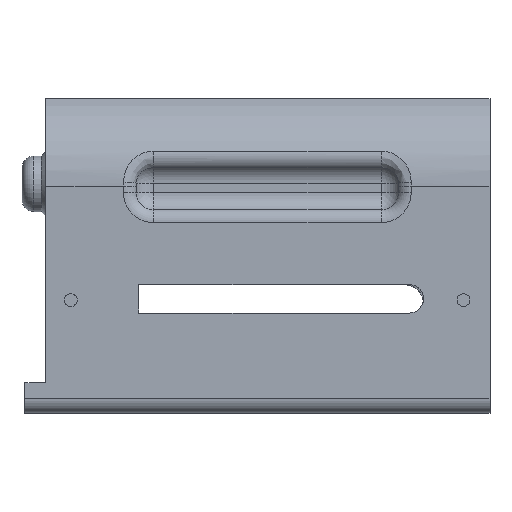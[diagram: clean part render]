
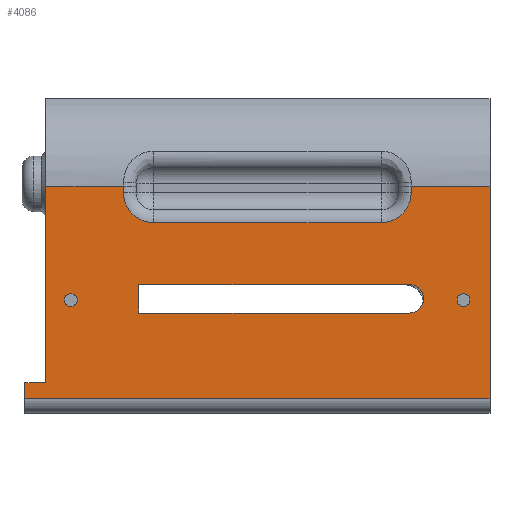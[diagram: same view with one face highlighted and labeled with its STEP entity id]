
A CAD part, top view. The second image highlights one B-rep face of the part: STEP entity #4086.
In plain terms, the highlighted planar face has unit normal (0, 0, 1).
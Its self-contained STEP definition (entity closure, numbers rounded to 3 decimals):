
#24 = ORIENTED_EDGE ( 'NONE', *, *, #6329, .F. ) ;
#39 = CARTESIAN_POINT ( 'NONE',  ( 83.403, 40.151, 20.1 ) ) ;
#65 = AXIS2_PLACEMENT_3D ( 'NONE', #5753, #6270, #804 ) ;
#95 = VERTEX_POINT ( 'NONE', #1609 ) ;
#123 = FACE_BOUND ( 'NONE', #307, .T. ) ;
#135 = LINE ( 'NONE', #2848, #3104 ) ;
#181 = VERTEX_POINT ( 'NONE', #1326 ) ;
#194 = LINE ( 'NONE', #2502, #4265 ) ;
#267 = VECTOR ( 'NONE', #2964, 1000. ) ;
#307 = EDGE_LOOP ( 'NONE', ( #24, #4251, #1701, #4105 ) ) ;
#310 = DIRECTION ( 'NONE',  ( -0.707, -0.707, 0. ) ) ;
#328 = CIRCLE ( 'NONE', #1395, 1.35 ) ;
#372 = EDGE_CURVE ( 'NONE', #4874, #4902, #4618, .T. ) ;
#436 = DIRECTION ( 'NONE',  ( 0., 0., 1. ) ) ;
#480 = CARTESIAN_POINT ( 'NONE',  ( 106.318, 71.272, 20.1 ) ) ;
#500 = VECTOR ( 'NONE', #5597, 1000. ) ;
#507 = CIRCLE ( 'NONE', #65, 6.325 ) ;
#534 = CARTESIAN_POINT ( 'NONE',  ( 17.987, 23.82, 20.1 ) ) ;
#618 = VERTEX_POINT ( 'NONE', #5741 ) ;
#677 = VERTEX_POINT ( 'NONE', #3186 ) ;
#678 = CIRCLE ( 'NONE', #3314, 6.325 ) ;
#804 = DIRECTION ( 'NONE',  ( 0.707, -0.707, 0. ) ) ;
#860 = EDGE_LOOP ( 'NONE', ( #1579 ) ) ;
#869 = CARTESIAN_POINT ( 'NONE',  ( 89.318, 27.078, 20.1 ) ) ;
#918 = EDGE_CURVE ( 'NONE', #4902, #1303, #1089, .T. ) ;
#957 = CARTESIAN_POINT ( 'NONE',  ( 8.3, 3.06, 20.1 ) ) ;
#1036 = DIRECTION ( 'NONE',  ( 0., 0., -1. ) ) ;
#1089 = CIRCLE ( 'NONE', #3141, 3. ) ;
#1100 = EDGE_CURVE ( 'NONE', #5980, #677, #2735, .T. ) ;
#1127 = ORIENTED_EDGE ( 'NONE', *, *, #5812, .T. ) ;
#1143 = VECTOR ( 'NONE', #2233, 1000. ) ;
#1180 = ORIENTED_EDGE ( 'NONE', *, *, #1100, .T. ) ;
#1276 = CARTESIAN_POINT ( 'NONE',  ( 35.403, 46.476, 20.1 ) ) ;
#1278 = VECTOR ( 'NONE', #5903, 1000. ) ;
#1286 = ORIENTED_EDGE ( 'NONE', *, *, #6173, .F. ) ;
#1298 = VERTEX_POINT ( 'NONE', #3364 ) ;
#1300 = CARTESIAN_POINT ( 'NONE',  ( 29.079, 47.476, 20.1 ) ) ;
#1303 = VERTEX_POINT ( 'NONE', #869 ) ;
#1326 = CARTESIAN_POINT ( 'NONE',  ( 16.637, 23.82, 20.1 ) ) ;
#1349 = VECTOR ( 'NONE', #4595, 1000. ) ;
#1395 = AXIS2_PLACEMENT_3D ( 'NONE', #534, #3577, #5480 ) ;
#1575 = DIRECTION ( 'NONE',  ( 0., 1., 0. ) ) ;
#1579 = ORIENTED_EDGE ( 'NONE', *, *, #5364, .T. ) ;
#1609 = CARTESIAN_POINT ( 'NONE',  ( 32.318, 27.078, 20.1 ) ) ;
#1679 = LINE ( 'NONE', #1300, #2920 ) ;
#1701 = ORIENTED_EDGE ( 'NONE', *, *, #918, .F. ) ;
#1733 = CARTESIAN_POINT ( 'NONE',  ( 12.7, 3.06, 20.1 ) ) ;
#1740 = CARTESIAN_POINT ( 'NONE',  ( 12.7, 6.41, 20.1 ) ) ;
#1744 = VERTEX_POINT ( 'NONE', #39 ) ;
#1795 = ORIENTED_EDGE ( 'NONE', *, *, #5772, .F. ) ;
#1825 = LINE ( 'NONE', #1995, #5494 ) ;
#1828 = CARTESIAN_POINT ( 'NONE',  ( 18.04, 47.837, 20.1 ) ) ;
#1995 = CARTESIAN_POINT ( 'NONE',  ( 89.728, 47.476, 20.1 ) ) ;
#2050 = VECTOR ( 'NONE', #5286, 1000. ) ;
#2138 = AXIS2_PLACEMENT_3D ( 'NONE', #6451, #2908, #1575 ) ;
#2212 = LINE ( 'NONE', #1828, #2050 ) ;
#2213 = EDGE_LOOP ( 'NONE', ( #3855 ) ) ;
#2233 = DIRECTION ( 'NONE',  ( -1., 0., 0. ) ) ;
#2243 = CARTESIAN_POINT ( 'NONE',  ( 8.3, 6.41, 20.1 ) ) ;
#2251 = VECTOR ( 'NONE', #3181, 1000. ) ;
#2276 = CARTESIAN_POINT ( 'NONE',  ( 32.318, 21.078, 20.1 ) ) ;
#2292 = CARTESIAN_POINT ( 'NONE',  ( 89.728, 46.476, 20.1 ) ) ;
#2496 = CARTESIAN_POINT ( 'NONE',  ( 32.318, 12.068, 20.1 ) ) ;
#2502 = CARTESIAN_POINT ( 'NONE',  ( 8.3, 45.001, 20.1 ) ) ;
#2638 = EDGE_CURVE ( 'NONE', #1303, #95, #135, .T. ) ;
#2689 = LINE ( 'NONE', #2496, #500 ) ;
#2735 = LINE ( 'NONE', #6049, #2251 ) ;
#2747 = ORIENTED_EDGE ( 'NONE', *, *, #5531, .F. ) ;
#2794 = CARTESIAN_POINT ( 'NONE',  ( 25.408, 21.078, 20.1 ) ) ;
#2820 = EDGE_CURVE ( 'NONE', #3206, #5874, #5272, .T. ) ;
#2835 = DIRECTION ( 'NONE',  ( 0., -1., 0. ) ) ;
#2848 = CARTESIAN_POINT ( 'NONE',  ( 25.408, 27.078, 20.1 ) ) ;
#2851 = LINE ( 'NONE', #480, #267 ) ;
#2908 = DIRECTION ( 'NONE',  ( 0., 0., -1. ) ) ;
#2916 = VERTEX_POINT ( 'NONE', #5376 ) ;
#2920 = VECTOR ( 'NONE', #2835, 1000. ) ;
#2960 = VERTEX_POINT ( 'NONE', #2243 ) ;
#2964 = DIRECTION ( 'NONE',  ( 0., 1., 0. ) ) ;
#3104 = VECTOR ( 'NONE', #4840, 1000. ) ;
#3141 = AXIS2_PLACEMENT_3D ( 'NONE', #4435, #436, #3921 ) ;
#3181 = DIRECTION ( 'NONE',  ( 0., -1., 0. ) ) ;
#3186 = CARTESIAN_POINT ( 'NONE',  ( 12.7, 6.41, 20.1 ) ) ;
#3206 = VERTEX_POINT ( 'NONE', #4051 ) ;
#3314 = AXIS2_PLACEMENT_3D ( 'NONE', #1276, #3316, #310 ) ;
#3316 = DIRECTION ( 'NONE',  ( 0., 0., 1. ) ) ;
#3332 = FACE_OUTER_BOUND ( 'NONE', #3971, .T. ) ;
#3364 = CARTESIAN_POINT ( 'NONE',  ( 35.403, 40.151, 20.1 ) ) ;
#3369 = CARTESIAN_POINT ( 'NONE',  ( 29.079, 47.837, 20.1 ) ) ;
#3406 = CARTESIAN_POINT ( 'NONE',  ( 89.728, 47.837, 20.1 ) ) ;
#3504 = EDGE_CURVE ( 'NONE', #618, #1298, #678, .T. ) ;
#3513 = ORIENTED_EDGE ( 'NONE', *, *, #6301, .F. ) ;
#3577 = DIRECTION ( 'NONE',  ( 0., 0., -1. ) ) ;
#3626 = ORIENTED_EDGE ( 'NONE', *, *, #5834, .T. ) ;
#3688 = CARTESIAN_POINT ( 'NONE',  ( 106.318, 47.837, 20.1 ) ) ;
#3796 = LINE ( 'NONE', #4507, #1278 ) ;
#3855 = ORIENTED_EDGE ( 'NONE', *, *, #5410, .T. ) ;
#3867 = CIRCLE ( 'NONE', #6321, 1.35 ) ;
#3921 = DIRECTION ( 'NONE',  ( 0.707, 0.707, 0. ) ) ;
#3928 = EDGE_CURVE ( 'NONE', #677, #2960, #4661, .T. ) ;
#3971 = EDGE_LOOP ( 'NONE', ( #1180, #5826, #1127, #5479, #3626, #2747, #3513, #4597, #1795, #5221, #4472, #1286 ) ) ;
#4002 = VERTEX_POINT ( 'NONE', #3369 ) ;
#4051 = CARTESIAN_POINT ( 'NONE',  ( 106.318, 3.06, 20.1 ) ) ;
#4086 = ADVANCED_FACE ( 'NONE', ( #3332, #5336, #4124, #123 ), #6361, .F. ) ;
#4105 = ORIENTED_EDGE ( 'NONE', *, *, #372, .F. ) ;
#4124 = FACE_BOUND ( 'NONE', #860, .T. ) ;
#4186 = LINE ( 'NONE', #5101, #1349 ) ;
#4251 = ORIENTED_EDGE ( 'NONE', *, *, #2638, .F. ) ;
#4254 = VERTEX_POINT ( 'NONE', #3688 ) ;
#4265 = VECTOR ( 'NONE', #5449, 1000. ) ;
#4435 = CARTESIAN_POINT ( 'NONE',  ( 89.318, 24.078, 20.1 ) ) ;
#4472 = ORIENTED_EDGE ( 'NONE', *, *, #4767, .F. ) ;
#4507 = CARTESIAN_POINT ( 'NONE',  ( 59.403, 40.151, 20.1 ) ) ;
#4551 = CARTESIAN_POINT ( 'NONE',  ( 12.7, 47.837, 20.1 ) ) ;
#4595 = DIRECTION ( 'NONE',  ( 1., 0., 0. ) ) ;
#4597 = ORIENTED_EDGE ( 'NONE', *, *, #4808, .F. ) ;
#4618 = LINE ( 'NONE', #2794, #5463 ) ;
#4661 = LINE ( 'NONE', #1740, #1143 ) ;
#4767 = EDGE_CURVE ( 'NONE', #4002, #618, #1679, .T. ) ;
#4808 = EDGE_CURVE ( 'NONE', #1744, #5191, #507, .T. ) ;
#4840 = DIRECTION ( 'NONE',  ( -1., 0., 0. ) ) ;
#4874 = VERTEX_POINT ( 'NONE', #2276 ) ;
#4902 = VERTEX_POINT ( 'NONE', #5856 ) ;
#4924 = VERTEX_POINT ( 'NONE', #3406 ) ;
#5101 = CARTESIAN_POINT ( 'NONE',  ( 18.04, 47.837, 20.1 ) ) ;
#5191 = VERTEX_POINT ( 'NONE', #2292 ) ;
#5221 = ORIENTED_EDGE ( 'NONE', *, *, #3504, .F. ) ;
#5270 = DIRECTION ( 'NONE',  ( 1., 0., 0. ) ) ;
#5272 = LINE ( 'NONE', #1733, #5429 ) ;
#5286 = DIRECTION ( 'NONE',  ( 1., 0., 0. ) ) ;
#5336 = FACE_BOUND ( 'NONE', #2213, .T. ) ;
#5364 = EDGE_CURVE ( 'NONE', #181, #181, #328, .T. ) ;
#5376 = CARTESIAN_POINT ( 'NONE',  ( 99.376, 23.82, 20.1 ) ) ;
#5410 = EDGE_CURVE ( 'NONE', #2916, #2916, #3867, .T. ) ;
#5429 = VECTOR ( 'NONE', #6156, 1000. ) ;
#5449 = DIRECTION ( 'NONE',  ( 0., -1., 0. ) ) ;
#5463 = VECTOR ( 'NONE', #5270, 1000. ) ;
#5479 = ORIENTED_EDGE ( 'NONE', *, *, #2820, .F. ) ;
#5480 = DIRECTION ( 'NONE',  ( -1., 0., 0. ) ) ;
#5494 = VECTOR ( 'NONE', #6104, 1000. ) ;
#5527 = DIRECTION ( 'NONE',  ( -1., 0., 0. ) ) ;
#5531 = EDGE_CURVE ( 'NONE', #4924, #4254, #4186, .T. ) ;
#5597 = DIRECTION ( 'NONE',  ( 0., -1., 0. ) ) ;
#5741 = CARTESIAN_POINT ( 'NONE',  ( 29.079, 46.476, 20.1 ) ) ;
#5753 = CARTESIAN_POINT ( 'NONE',  ( 83.403, 46.476, 20.1 ) ) ;
#5772 = EDGE_CURVE ( 'NONE', #1298, #1744, #3796, .T. ) ;
#5812 = EDGE_CURVE ( 'NONE', #2960, #5874, #194, .T. ) ;
#5826 = ORIENTED_EDGE ( 'NONE', *, *, #3928, .T. ) ;
#5834 = EDGE_CURVE ( 'NONE', #3206, #4254, #2851, .T. ) ;
#5856 = CARTESIAN_POINT ( 'NONE',  ( 89.318, 21.078, 20.1 ) ) ;
#5874 = VERTEX_POINT ( 'NONE', #957 ) ;
#5903 = DIRECTION ( 'NONE',  ( 1., 0., 0. ) ) ;
#5980 = VERTEX_POINT ( 'NONE', #4551 ) ;
#6028 = CARTESIAN_POINT ( 'NONE',  ( 100.726, 23.82, 20.1 ) ) ;
#6049 = CARTESIAN_POINT ( 'NONE',  ( 12.7, 60.786, 20.1 ) ) ;
#6104 = DIRECTION ( 'NONE',  ( 0., 1., 0. ) ) ;
#6156 = DIRECTION ( 'NONE',  ( -1., 0., 0. ) ) ;
#6173 = EDGE_CURVE ( 'NONE', #5980, #4002, #2212, .T. ) ;
#6270 = DIRECTION ( 'NONE',  ( 0., 0., 1. ) ) ;
#6301 = EDGE_CURVE ( 'NONE', #5191, #4924, #1825, .T. ) ;
#6321 = AXIS2_PLACEMENT_3D ( 'NONE', #6028, #1036, #5527 ) ;
#6329 = EDGE_CURVE ( 'NONE', #95, #4874, #2689, .T. ) ;
#6361 = PLANE ( 'NONE',  #2138 ) ;
#6451 = CARTESIAN_POINT ( 'NONE',  ( 5.499, 0.058, 20.1 ) ) ;
